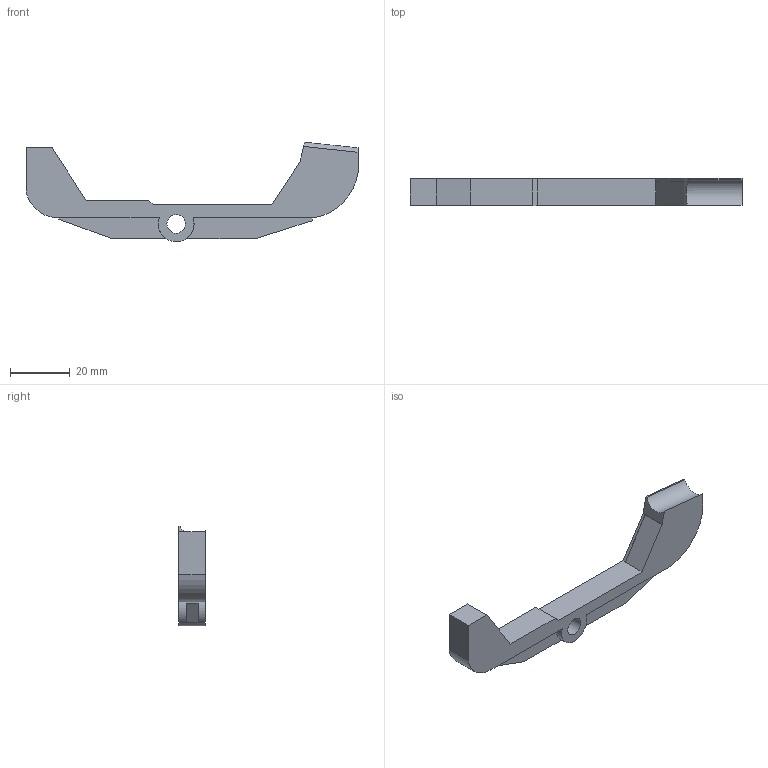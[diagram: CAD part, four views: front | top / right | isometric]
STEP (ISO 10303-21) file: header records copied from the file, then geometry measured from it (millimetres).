
FILE_DESCRIPTION (( 'STEP AP203' ), '1' );
FILE_NAME ('WTF-9_hillbilly_ejector.STEP', '2020-05-09T08:57:15', ( '' ), ( '' ), 'SwSTEP 2.0', 'SolidWorks 2016', '' );
FILE_SCHEMA (( 'CONFIG_CONTROL_DESIGN' ));
Length unit declared in the file: millimetre
Products named in the file (2): WTF HILLBILLY FINAL_3; WTF-9_hillbilly_ejector
Assembly tree (1 placements, depth 2):
  WTF-9_hillbilly_ejector
    WTF HILLBILLY FINAL_3
Bounding box: 111.36 x 9.05 x 33.41 mm (x, y, z)
Volume: 12307.2 mm3; surface area: 6026.7 mm2
Topology: 1 solids, 1 shells, 36 faces, 101 edges, 67 vertices
Faces by surface type: plane 31, cylinder 5
Full cylindrical faces by diameter (mm): 6.2 x1
Entity records: 1344 total; most frequent: CARTESIAN_POINT 216, ORIENTED_EDGE 200, DIRECTION 189, EDGE_CURVE 100, LINE 85, VECTOR 85, VERTEX_POINT 67, AXIS2_PLACEMENT_3D 52
